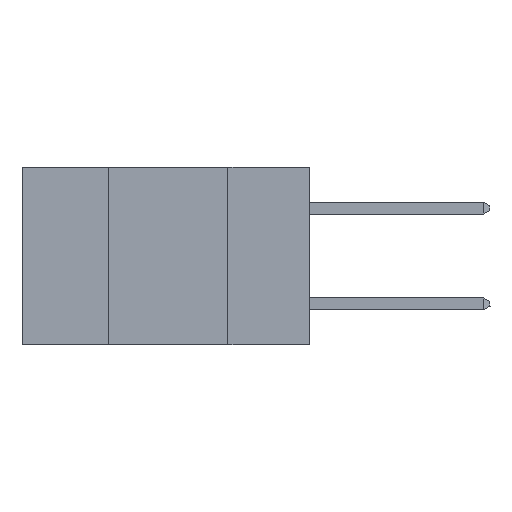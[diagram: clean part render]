
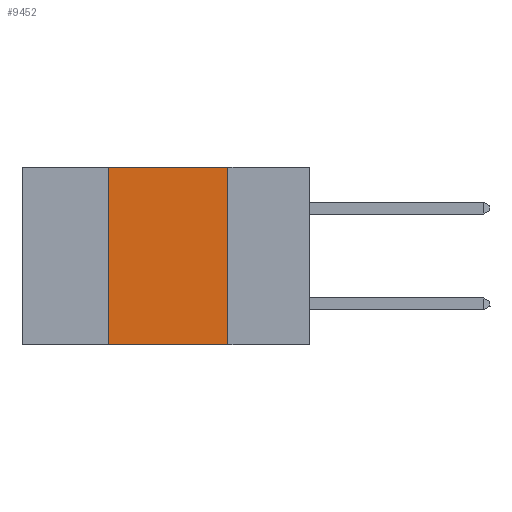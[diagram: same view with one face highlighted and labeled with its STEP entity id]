
A CAD part, left-side view. The second image highlights one B-rep face of the part: STEP entity #9452.
In plain terms, the highlighted planar face has unit normal (-1, 0, 0).
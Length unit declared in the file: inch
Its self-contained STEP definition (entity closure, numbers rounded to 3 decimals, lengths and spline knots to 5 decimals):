
#600 = CARTESIAN_POINT ( 'NONE',  ( 0., 0.42, 0. ) ) ;
#906 = CARTESIAN_POINT ( 'NONE',  ( 0., 0.6, 0. ) ) ;
#2368 = DIRECTION ( 'NONE',  ( 0., 0., -1. ) ) ;
#2650 = CARTESIAN_POINT ( 'NONE',  ( 0., 0.17, -0.37 ) ) ;
#2660 = VERTEX_POINT ( 'NONE', #6999 ) ;
#2813 = DIRECTION ( 'NONE',  ( 0., 0., 1. ) ) ;
#3403 = CARTESIAN_POINT ( 'NONE',  ( 0., 0.6, 0. ) ) ;
#3620 = ORIENTED_EDGE ( 'NONE', *, *, #6031, .F. ) ;
#4297 = ORIENTED_EDGE ( 'NONE', *, *, #6735, .F. ) ;
#4435 = VECTOR ( 'NONE', #2813, 39.37008 ) ;
#4992 = CARTESIAN_POINT ( 'NONE',  ( 0., 0.42, 0. ) ) ;
#5372 = VERTEX_POINT ( 'NONE', #2650 ) ;
#5511 = LINE ( 'NONE', #8358, #8050 ) ;
#6031 = EDGE_CURVE ( 'NONE', #2660, #5372, #12055, .T. ) ;
#6057 = DIRECTION ( 'NONE',  ( 0., 0., -1. ) ) ;
#6732 = PLANE ( 'NONE',  #12003 ) ;
#6735 = EDGE_CURVE ( 'NONE', #9816, #6803, #7314, .T. ) ;
#6803 = VERTEX_POINT ( 'NONE', #600 ) ;
#6999 = CARTESIAN_POINT ( 'NONE',  ( 0., 0.17, 0. ) ) ;
#7142 = CARTESIAN_POINT ( 'NONE',  ( 0., 0.17, 0. ) ) ;
#7314 = LINE ( 'NONE', #4992, #4435 ) ;
#8050 = VECTOR ( 'NONE', #12613, 39.37008 ) ;
#8358 = CARTESIAN_POINT ( 'NONE',  ( 0., 0.6, -0.37 ) ) ;
#8429 = CARTESIAN_POINT ( 'NONE',  ( 0., 0.42, -0.37 ) ) ;
#8541 = VECTOR ( 'NONE', #6057, 39.37008 ) ;
#8922 = DIRECTION ( 'NONE',  ( 1., 0., 0. ) ) ;
#9452 = ADVANCED_FACE ( 'NONE', ( #12919 ), #6732, .F. ) ;
#9740 = ORIENTED_EDGE ( 'NONE', *, *, #9957, .F. ) ;
#9774 = VECTOR ( 'NONE', #11838, 39.37008 ) ;
#9816 = VERTEX_POINT ( 'NONE', #8429 ) ;
#9957 = EDGE_CURVE ( 'NONE', #6803, #2660, #10774, .T. ) ;
#10569 = EDGE_CURVE ( 'NONE', #9816, #5372, #5511, .T. ) ;
#10774 = LINE ( 'NONE', #906, #9774 ) ;
#11283 = EDGE_LOOP ( 'NONE', ( #3620, #9740, #4297, #13210 ) ) ;
#11838 = DIRECTION ( 'NONE',  ( 0., -1., 0. ) ) ;
#12003 = AXIS2_PLACEMENT_3D ( 'NONE', #3403, #8922, #2368 ) ;
#12055 = LINE ( 'NONE', #7142, #8541 ) ;
#12613 = DIRECTION ( 'NONE',  ( 0., -1., 0. ) ) ;
#12919 = FACE_OUTER_BOUND ( 'NONE', #11283, .T. ) ;
#13210 = ORIENTED_EDGE ( 'NONE', *, *, #10569, .T. ) ;
